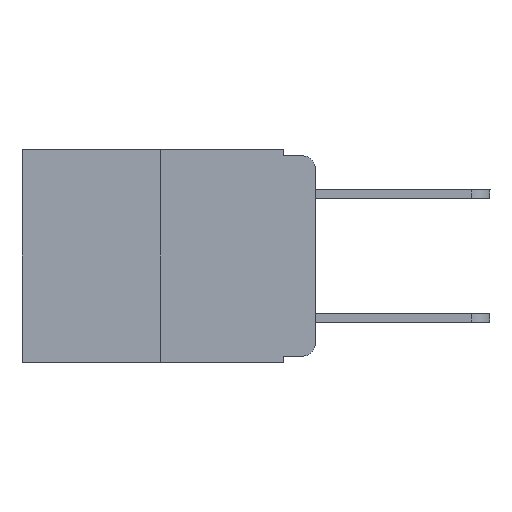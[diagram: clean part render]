
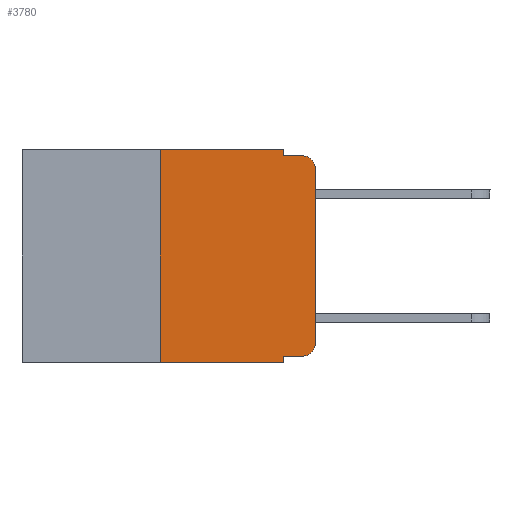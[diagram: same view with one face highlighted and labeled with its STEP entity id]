
A CAD part, left-side view. The second image highlights one B-rep face of the part: STEP entity #3780.
In plain terms, the highlighted planar face has unit normal (-1, 0, 0).
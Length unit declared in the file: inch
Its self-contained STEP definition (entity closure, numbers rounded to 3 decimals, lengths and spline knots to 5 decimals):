
#56 = LINE ( 'NONE', #4219, #884 ) ;
#119 = EDGE_CURVE ( 'NONE', #9560, #6728, #2583, .T. ) ;
#121 = ORIENTED_EDGE ( 'NONE', *, *, #4745, .T. ) ;
#335 = EDGE_CURVE ( 'NONE', #13297, #6728, #7941, .T. ) ;
#368 = CARTESIAN_POINT ( 'NONE',  ( 0., 0.051, -0.01 ) ) ;
#475 = EDGE_CURVE ( 'NONE', #5142, #1306, #12475, .T. ) ;
#884 = VECTOR ( 'NONE', #8431, 39.37008 ) ;
#896 = CARTESIAN_POINT ( 'NONE',  ( 0., 0.051, -0.333 ) ) ;
#949 = EDGE_CURVE ( 'NONE', #5142, #10833, #13420, .T. ) ;
#1099 = ORIENTED_EDGE ( 'NONE', *, *, #475, .T. ) ;
#1306 = VERTEX_POINT ( 'NONE', #11369 ) ;
#1427 = ORIENTED_EDGE ( 'NONE', *, *, #13467, .F. ) ;
#1987 = VECTOR ( 'NONE', #11537, 39.37008 ) ;
#2369 = DIRECTION ( 'NONE',  ( -1., 0., 0. ) ) ;
#2490 = EDGE_CURVE ( 'NONE', #9206, #10833, #12790, .T. ) ;
#2583 = CIRCLE ( 'NONE', #12030, 0.02 ) ;
#2955 = LINE ( 'NONE', #13230, #3836 ) ;
#3036 = CARTESIAN_POINT ( 'NONE',  ( 0., 0.051, -0.333 ) ) ;
#3268 = ORIENTED_EDGE ( 'NONE', *, *, #8459, .F. ) ;
#3780 = ADVANCED_FACE ( 'NONE', ( #8174 ), #10375, .F. ) ;
#3836 = VECTOR ( 'NONE', #10060, 39.37008 ) ;
#3845 = VECTOR ( 'NONE', #3855, 39.37008 ) ;
#3855 = DIRECTION ( 'NONE',  ( 0., -1., 0. ) ) ;
#3918 = CARTESIAN_POINT ( 'NONE',  ( 0., 0.25, -0.343 ) ) ;
#4042 = CARTESIAN_POINT ( 'NONE',  ( 0., 0., 0. ) ) ;
#4219 = CARTESIAN_POINT ( 'NONE',  ( 0., 0.25, 0. ) ) ;
#4494 = VECTOR ( 'NONE', #11075, 39.37008 ) ;
#4597 = LINE ( 'NONE', #9078, #5946 ) ;
#4745 = EDGE_CURVE ( 'NONE', #1306, #9489, #9627, .T. ) ;
#5142 = VERTEX_POINT ( 'NONE', #896 ) ;
#5566 = CARTESIAN_POINT ( 'NONE',  ( 0., 0.02, -0.01 ) ) ;
#5946 = VECTOR ( 'NONE', #6688, 39.37008 ) ;
#5973 = VERTEX_POINT ( 'NONE', #10339 ) ;
#6213 = EDGE_CURVE ( 'NONE', #9489, #9560, #7104, .T. ) ;
#6344 = ORIENTED_EDGE ( 'NONE', *, *, #335, .F. ) ;
#6360 = EDGE_LOOP ( 'NONE', ( #12574, #12043, #6344, #7962, #1427, #3268, #12183, #10853, #1099, #121 ) ) ;
#6688 = DIRECTION ( 'NONE',  ( 0., 0., -1. ) ) ;
#6728 = VERTEX_POINT ( 'NONE', #5566 ) ;
#6969 = CARTESIAN_POINT ( 'NONE',  ( 0., 0., -0.03 ) ) ;
#7050 = CARTESIAN_POINT ( 'NONE',  ( 0., 0.02, -0.313 ) ) ;
#7092 = DIRECTION ( 'NONE',  ( 0., 0., -1. ) ) ;
#7104 = LINE ( 'NONE', #4042, #1987 ) ;
#7217 = AXIS2_PLACEMENT_3D ( 'NONE', #7050, #8200, #12408 ) ;
#7491 = CARTESIAN_POINT ( 'NONE',  ( 0., 0.473, -0.343 ) ) ;
#7728 = CARTESIAN_POINT ( 'NONE',  ( 0., 0., -0.313 ) ) ;
#7941 = LINE ( 'NONE', #12129, #4494 ) ;
#7962 = ORIENTED_EDGE ( 'NONE', *, *, #9999, .F. ) ;
#8174 = FACE_OUTER_BOUND ( 'NONE', #6360, .T. ) ;
#8178 = VECTOR ( 'NONE', #9544, 39.37008 ) ;
#8200 = DIRECTION ( 'NONE',  ( -1., 0., 0. ) ) ;
#8431 = DIRECTION ( 'NONE',  ( 0., 0., 1. ) ) ;
#8459 = EDGE_CURVE ( 'NONE', #9206, #5973, #56, .T. ) ;
#9078 = CARTESIAN_POINT ( 'NONE',  ( 0., 0.051, 0. ) ) ;
#9206 = VERTEX_POINT ( 'NONE', #3918 ) ;
#9489 = VERTEX_POINT ( 'NONE', #7728 ) ;
#9544 = DIRECTION ( 'NONE',  ( 0., -1., 0. ) ) ;
#9560 = VERTEX_POINT ( 'NONE', #6969 ) ;
#9627 = CIRCLE ( 'NONE', #7217, 0.02 ) ;
#9999 = EDGE_CURVE ( 'NONE', #13190, #13297, #4597, .T. ) ;
#10060 = DIRECTION ( 'NONE',  ( 0., -1., 0. ) ) ;
#10234 = CARTESIAN_POINT ( 'NONE',  ( 0., 0.473, 0. ) ) ;
#10339 = CARTESIAN_POINT ( 'NONE',  ( 0., 0.25, 0. ) ) ;
#10375 = PLANE ( 'NONE',  #11110 ) ;
#10508 = DIRECTION ( 'NONE',  ( 1., 0., 0. ) ) ;
#10650 = VECTOR ( 'NONE', #12315, 39.37008 ) ;
#10833 = VERTEX_POINT ( 'NONE', #11456 ) ;
#10853 = ORIENTED_EDGE ( 'NONE', *, *, #949, .F. ) ;
#11075 = DIRECTION ( 'NONE',  ( 0., -1., 0. ) ) ;
#11110 = AXIS2_PLACEMENT_3D ( 'NONE', #10234, #10508, #7092 ) ;
#11194 = CARTESIAN_POINT ( 'NONE',  ( 0., 0.051, 0. ) ) ;
#11369 = CARTESIAN_POINT ( 'NONE',  ( 0., 0.02, -0.333 ) ) ;
#11456 = CARTESIAN_POINT ( 'NONE',  ( 0., 0.051, -0.343 ) ) ;
#11492 = CARTESIAN_POINT ( 'NONE',  ( 0., 0.051, 0. ) ) ;
#11537 = DIRECTION ( 'NONE',  ( 0., 0., 1. ) ) ;
#11711 = DIRECTION ( 'NONE',  ( 0., 0., -1. ) ) ;
#12030 = AXIS2_PLACEMENT_3D ( 'NONE', #12900, #2369, #11711 ) ;
#12043 = ORIENTED_EDGE ( 'NONE', *, *, #119, .T. ) ;
#12129 = CARTESIAN_POINT ( 'NONE',  ( 0., 0.051, -0.01 ) ) ;
#12183 = ORIENTED_EDGE ( 'NONE', *, *, #2490, .T. ) ;
#12315 = DIRECTION ( 'NONE',  ( 0., 0., -1. ) ) ;
#12408 = DIRECTION ( 'NONE',  ( 0., 0., -1. ) ) ;
#12475 = LINE ( 'NONE', #3036, #3845 ) ;
#12574 = ORIENTED_EDGE ( 'NONE', *, *, #6213, .T. ) ;
#12790 = LINE ( 'NONE', #7491, #8178 ) ;
#12900 = CARTESIAN_POINT ( 'NONE',  ( 0., 0.02, -0.03 ) ) ;
#13190 = VERTEX_POINT ( 'NONE', #11492 ) ;
#13230 = CARTESIAN_POINT ( 'NONE',  ( 0., 0.473, 0. ) ) ;
#13297 = VERTEX_POINT ( 'NONE', #368 ) ;
#13420 = LINE ( 'NONE', #11194, #10650 ) ;
#13467 = EDGE_CURVE ( 'NONE', #5973, #13190, #2955, .T. ) ;
